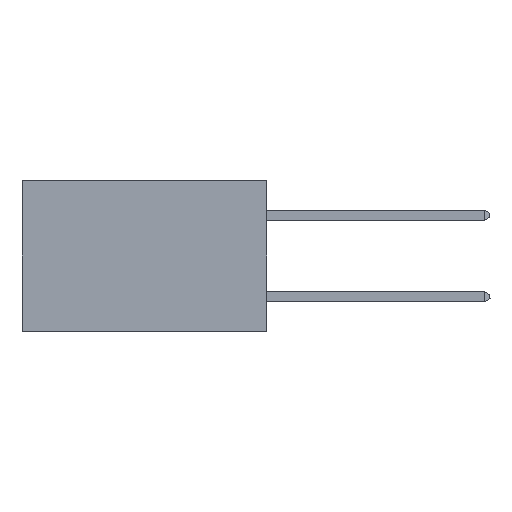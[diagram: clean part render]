
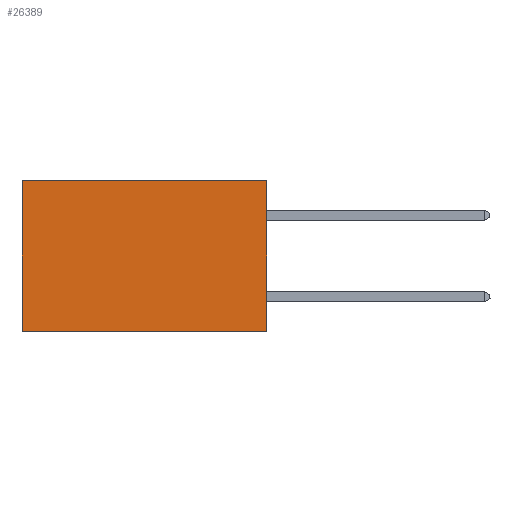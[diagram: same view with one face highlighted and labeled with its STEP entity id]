
A CAD part, left-side view. The second image highlights one B-rep face of the part: STEP entity #26389.
In plain terms, the highlighted planar face has unit normal (-1, 0, 0).
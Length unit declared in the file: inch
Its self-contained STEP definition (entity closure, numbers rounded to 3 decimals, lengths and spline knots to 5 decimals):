
#53 = VERTEX_POINT ( 'NONE', #38512 ) ;
#813 = VECTOR ( 'NONE', #15808, 39.37008 ) ;
#1768 = LINE ( 'NONE', #33497, #26860 ) ;
#3736 = DIRECTION ( 'NONE',  ( 0., 1., 0. ) ) ;
#3886 = CARTESIAN_POINT ( 'NONE',  ( 0.2875, 0.6, -0.37 ) ) ;
#4834 = VECTOR ( 'NONE', #14223, 39.37008 ) ;
#5575 = VERTEX_POINT ( 'NONE', #39137 ) ;
#5907 = CARTESIAN_POINT ( 'NONE',  ( 0.2875, 0., 0. ) ) ;
#6766 = LINE ( 'NONE', #38315, #4834 ) ;
#7433 = VECTOR ( 'NONE', #11113, 39.37008 ) ;
#7441 = EDGE_CURVE ( 'NONE', #53, #29968, #24943, .T. ) ;
#8344 = ORIENTED_EDGE ( 'NONE', *, *, #30363, .F. ) ;
#9313 = LINE ( 'NONE', #20367, #7433 ) ;
#10152 = VERTEX_POINT ( 'NONE', #3886 ) ;
#11113 = DIRECTION ( 'NONE',  ( 0., 0., -1. ) ) ;
#14223 = DIRECTION ( 'NONE',  ( 0., 1., 0. ) ) ;
#15265 = PLANE ( 'NONE',  #15534 ) ;
#15534 = AXIS2_PLACEMENT_3D ( 'NONE', #5907, #24498, #18421 ) ;
#15808 = DIRECTION ( 'NONE',  ( 0., 0., -1. ) ) ;
#16286 = EDGE_CURVE ( 'NONE', #53, #5575, #1768, .T. ) ;
#17697 = CARTESIAN_POINT ( 'NONE',  ( 0.2875, 0., 0. ) ) ;
#18421 = DIRECTION ( 'NONE',  ( 0., 0., -1. ) ) ;
#18434 = FACE_OUTER_BOUND ( 'NONE', #26643, .T. ) ;
#20312 = ORIENTED_EDGE ( 'NONE', *, *, #16286, .T. ) ;
#20367 = CARTESIAN_POINT ( 'NONE',  ( 0.2875, 0.6, 0. ) ) ;
#22196 = ORIENTED_EDGE ( 'NONE', *, *, #7441, .F. ) ;
#24498 = DIRECTION ( 'NONE',  ( 1., 0., 0. ) ) ;
#24943 = LINE ( 'NONE', #17697, #813 ) ;
#26389 = ADVANCED_FACE ( 'NONE', ( #18434 ), #15265, .F. ) ;
#26643 = EDGE_LOOP ( 'NONE', ( #33717, #8344, #22196, #20312 ) ) ;
#26860 = VECTOR ( 'NONE', #3736, 39.37008 ) ;
#29968 = VERTEX_POINT ( 'NONE', #32002 ) ;
#30363 = EDGE_CURVE ( 'NONE', #29968, #10152, #6766, .T. ) ;
#32002 = CARTESIAN_POINT ( 'NONE',  ( 0.2875, 0., -0.37 ) ) ;
#33497 = CARTESIAN_POINT ( 'NONE',  ( 0.2875, 0., 0. ) ) ;
#33717 = ORIENTED_EDGE ( 'NONE', *, *, #37983, .T. ) ;
#37983 = EDGE_CURVE ( 'NONE', #5575, #10152, #9313, .T. ) ;
#38315 = CARTESIAN_POINT ( 'NONE',  ( 0.2875, 0., -0.37 ) ) ;
#38512 = CARTESIAN_POINT ( 'NONE',  ( 0.2875, 0., 0. ) ) ;
#39137 = CARTESIAN_POINT ( 'NONE',  ( 0.2875, 0.6, 0. ) ) ;
